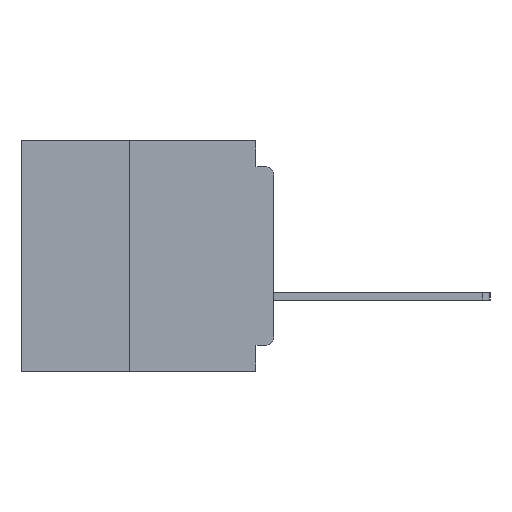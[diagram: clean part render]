
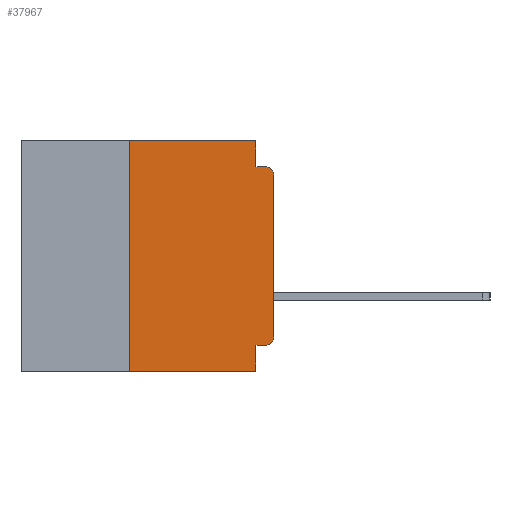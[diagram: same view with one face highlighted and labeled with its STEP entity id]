
A CAD part, left-side view. The second image highlights one B-rep face of the part: STEP entity #37967.
In plain terms, the highlighted planar face has unit normal (-1, 0, 0).
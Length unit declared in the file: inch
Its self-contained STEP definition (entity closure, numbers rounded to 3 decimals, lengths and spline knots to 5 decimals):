
#176 = ORIENTED_EDGE ( 'NONE', *, *, #34662, .T. ) ;
#810 = DIRECTION ( 'NONE',  ( 0., 0., -1. ) ) ;
#1218 = EDGE_CURVE ( 'NONE', #30355, #5235, #29416, .T. ) ;
#2520 = EDGE_LOOP ( 'NONE', ( #29947, #10365, #32427, #18037, #2585, #32714, #24578, #15135, #35775, #176 ) ) ;
#2585 = ORIENTED_EDGE ( 'NONE', *, *, #1218, .F. ) ;
#3133 = AXIS2_PLACEMENT_3D ( 'NONE', #36871, #18953, #810 ) ;
#3369 = VECTOR ( 'NONE', #7120, 39.37008 ) ;
#5235 = VERTEX_POINT ( 'NONE', #36994 ) ;
#5503 = DIRECTION ( 'NONE',  ( -1., 0., 0. ) ) ;
#5609 = DIRECTION ( 'NONE',  ( 0., -1., 0. ) ) ;
#5807 = VERTEX_POINT ( 'NONE', #21686 ) ;
#5848 = DIRECTION ( 'NONE',  ( 0., 0., 1. ) ) ;
#5956 = VERTEX_POINT ( 'NONE', #34454 ) ;
#6215 = CARTESIAN_POINT ( 'NONE',  ( 0., 0.031, -0.4 ) ) ;
#6311 = VECTOR ( 'NONE', #22045, 39.37008 ) ;
#6935 = VECTOR ( 'NONE', #5848, 39.37008 ) ;
#7120 = DIRECTION ( 'NONE',  ( 0., 0., -1. ) ) ;
#7474 = VERTEX_POINT ( 'NONE', #30711 ) ;
#7971 = DIRECTION ( 'NONE',  ( 0., -1., 0. ) ) ;
#8074 = AXIS2_PLACEMENT_3D ( 'NONE', #23578, #5503, #26600 ) ;
#8869 = CARTESIAN_POINT ( 'NONE',  ( 0., 0.25, 0. ) ) ;
#10365 = ORIENTED_EDGE ( 'NONE', *, *, #11857, .T. ) ;
#10746 = LINE ( 'NONE', #18127, #38026 ) ;
#10748 = EDGE_CURVE ( 'NONE', #38307, #30355, #10746, .T. ) ;
#11252 = DIRECTION ( 'NONE',  ( -1., 0., 0. ) ) ;
#11391 = VECTOR ( 'NONE', #5609, 39.37008 ) ;
#11754 = EDGE_CURVE ( 'NONE', #18773, #5807, #35849, .T. ) ;
#11857 = EDGE_CURVE ( 'NONE', #7474, #5956, #17108, .T. ) ;
#12336 = LINE ( 'NONE', #29717, #11391 ) ;
#12482 = FACE_OUTER_BOUND ( 'NONE', #2520, .T. ) ;
#13159 = VERTEX_POINT ( 'NONE', #6215 ) ;
#13196 = LINE ( 'NONE', #22181, #3369 ) ;
#15135 = ORIENTED_EDGE ( 'NONE', *, *, #27628, .F. ) ;
#15581 = VERTEX_POINT ( 'NONE', #18779 ) ;
#15968 = CARTESIAN_POINT ( 'NONE',  ( 0., 0.437, 0. ) ) ;
#17108 = CIRCLE ( 'NONE', #19919, 0.015 ) ;
#17396 = VECTOR ( 'NONE', #19787, 39.37008 ) ;
#18037 = ORIENTED_EDGE ( 'NONE', *, *, #31140, .F. ) ;
#18127 = CARTESIAN_POINT ( 'NONE',  ( 0., 0.25, -0.4 ) ) ;
#18263 = DIRECTION ( 'NONE',  ( 0., 0., 1. ) ) ;
#18773 = VERTEX_POINT ( 'NONE', #28985 ) ;
#18779 = CARTESIAN_POINT ( 'NONE',  ( 0., 0., -0.34 ) ) ;
#18953 = DIRECTION ( 'NONE',  ( 1., 0., 0. ) ) ;
#18959 = VECTOR ( 'NONE', #7971, 39.37008 ) ;
#19787 = DIRECTION ( 'NONE',  ( 0., 0., -1. ) ) ;
#19908 = DIRECTION ( 'NONE',  ( 0., 1., 0. ) ) ;
#19919 = AXIS2_PLACEMENT_3D ( 'NONE', #29368, #11252, #32356 ) ;
#20021 = CARTESIAN_POINT ( 'NONE',  ( 0., 0., -0.045 ) ) ;
#20919 = CARTESIAN_POINT ( 'NONE',  ( 0., 0., 0. ) ) ;
#21686 = CARTESIAN_POINT ( 'NONE',  ( 0., 0.031, -0.355 ) ) ;
#21771 = EDGE_CURVE ( 'NONE', #15581, #7474, #37933, .T. ) ;
#22045 = DIRECTION ( 'NONE',  ( 0., -1., 0. ) ) ;
#22181 = CARTESIAN_POINT ( 'NONE',  ( 0., 0.031, 0. ) ) ;
#23578 = CARTESIAN_POINT ( 'NONE',  ( 0., 0.015, -0.34 ) ) ;
#24578 = ORIENTED_EDGE ( 'NONE', *, *, #30292, .T. ) ;
#24997 = EDGE_CURVE ( 'NONE', #32942, #5956, #34879, .T. ) ;
#25853 = CARTESIAN_POINT ( 'NONE',  ( 0., 0., -0.355 ) ) ;
#26600 = DIRECTION ( 'NONE',  ( 0., 0., -1. ) ) ;
#27628 = EDGE_CURVE ( 'NONE', #5807, #13159, #33350, .T. ) ;
#27955 = VECTOR ( 'NONE', #19908, 39.37008 ) ;
#28985 = CARTESIAN_POINT ( 'NONE',  ( 0., 0.015, -0.355 ) ) ;
#29368 = CARTESIAN_POINT ( 'NONE',  ( 0., 0.015, -0.06 ) ) ;
#29416 = LINE ( 'NONE', #15968, #6311 ) ;
#29452 = CARTESIAN_POINT ( 'NONE',  ( 0., 0.25, -0.4 ) ) ;
#29717 = CARTESIAN_POINT ( 'NONE',  ( 0., 0.437, -0.4 ) ) ;
#29947 = ORIENTED_EDGE ( 'NONE', *, *, #21771, .T. ) ;
#30292 = EDGE_CURVE ( 'NONE', #38307, #13159, #12336, .T. ) ;
#30355 = VERTEX_POINT ( 'NONE', #8869 ) ;
#30711 = CARTESIAN_POINT ( 'NONE',  ( 0., 0., -0.06 ) ) ;
#30894 = PLANE ( 'NONE',  #3133 ) ;
#31140 = EDGE_CURVE ( 'NONE', #5235, #32942, #13196, .T. ) ;
#31845 = CIRCLE ( 'NONE', #8074, 0.015 ) ;
#32356 = DIRECTION ( 'NONE',  ( 0., 0., -1. ) ) ;
#32427 = ORIENTED_EDGE ( 'NONE', *, *, #24997, .F. ) ;
#32714 = ORIENTED_EDGE ( 'NONE', *, *, #10748, .F. ) ;
#32942 = VERTEX_POINT ( 'NONE', #36793 ) ;
#33350 = LINE ( 'NONE', #34696, #17396 ) ;
#34454 = CARTESIAN_POINT ( 'NONE',  ( 0., 0.015, -0.045 ) ) ;
#34662 = EDGE_CURVE ( 'NONE', #18773, #15581, #31845, .T. ) ;
#34696 = CARTESIAN_POINT ( 'NONE',  ( 0., 0.031, -0.4 ) ) ;
#34879 = LINE ( 'NONE', #20021, #18959 ) ;
#35775 = ORIENTED_EDGE ( 'NONE', *, *, #11754, .F. ) ;
#35849 = LINE ( 'NONE', #25853, #27955 ) ;
#36793 = CARTESIAN_POINT ( 'NONE',  ( 0., 0.031, -0.045 ) ) ;
#36871 = CARTESIAN_POINT ( 'NONE',  ( 0., 0.437, 0. ) ) ;
#36994 = CARTESIAN_POINT ( 'NONE',  ( 0., 0.031, 0. ) ) ;
#37933 = LINE ( 'NONE', #20919, #6935 ) ;
#37967 = ADVANCED_FACE ( 'NONE', ( #12482 ), #30894, .F. ) ;
#38026 = VECTOR ( 'NONE', #18263, 39.37008 ) ;
#38307 = VERTEX_POINT ( 'NONE', #29452 ) ;
